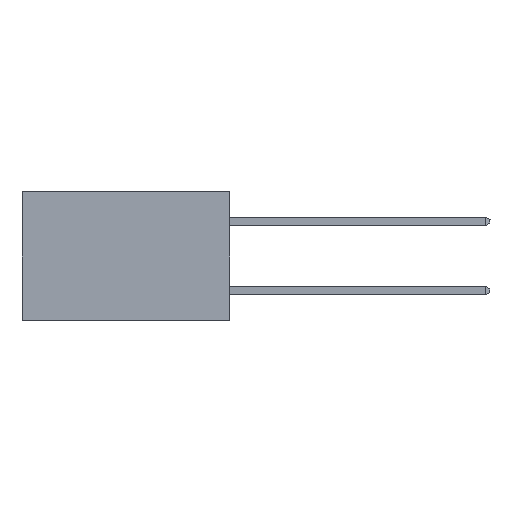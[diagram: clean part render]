
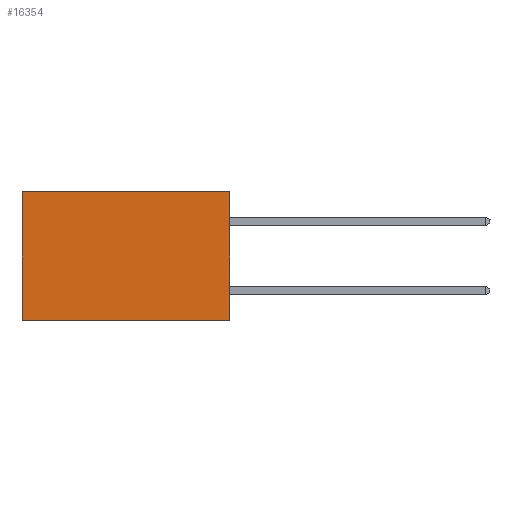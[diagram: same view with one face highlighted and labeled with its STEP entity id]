
A CAD part, left-side view. The second image highlights one B-rep face of the part: STEP entity #16354.
In plain terms, the highlighted planar face has unit normal (-1, 0, 0).
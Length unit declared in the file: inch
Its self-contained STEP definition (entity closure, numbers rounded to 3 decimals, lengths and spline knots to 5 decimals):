
#354 = CARTESIAN_POINT ( 'NONE',  ( 0.2615, 0., -0.37 ) ) ;
#1392 = FACE_OUTER_BOUND ( 'NONE', #18356, .T. ) ;
#1597 = VERTEX_POINT ( 'NONE', #5173 ) ;
#2340 = LINE ( 'NONE', #4180, #2395 ) ;
#2395 = VECTOR ( 'NONE', #3834, 39.37008 ) ;
#3674 = DIRECTION ( 'NONE',  ( 0., 0., -1. ) ) ;
#3834 = DIRECTION ( 'NONE',  ( 0., 0., -1. ) ) ;
#4180 = CARTESIAN_POINT ( 'NONE',  ( 0.2615, 0., -0.37 ) ) ;
#5068 = CARTESIAN_POINT ( 'NONE',  ( 0.2615, 0.6, -0.37 ) ) ;
#5173 = CARTESIAN_POINT ( 'NONE',  ( 0.2615, 0., -0.37 ) ) ;
#7219 = AXIS2_PLACEMENT_3D ( 'NONE', #8432, #11876, #11768 ) ;
#7254 = LINE ( 'NONE', #20901, #11094 ) ;
#8432 = CARTESIAN_POINT ( 'NONE',  ( 0.2615, 0., -0.37 ) ) ;
#8783 = EDGE_CURVE ( 'NONE', #10964, #18353, #7254, .T. ) ;
#9097 = LINE ( 'NONE', #354, #11551 ) ;
#10845 = CARTESIAN_POINT ( 'NONE',  ( 0.2615, 0., 0. ) ) ;
#10964 = VERTEX_POINT ( 'NONE', #17326 ) ;
#11094 = VECTOR ( 'NONE', #3674, 39.37008 ) ;
#11463 = ORIENTED_EDGE ( 'NONE', *, *, #13943, .T. ) ;
#11514 = ORIENTED_EDGE ( 'NONE', *, *, #13380, .F. ) ;
#11551 = VECTOR ( 'NONE', #14171, 39.37008 ) ;
#11586 = CARTESIAN_POINT ( 'NONE',  ( 0.2615, 0., 0. ) ) ;
#11768 = DIRECTION ( 'NONE',  ( 0., 0., -1. ) ) ;
#11876 = DIRECTION ( 'NONE',  ( 1., 0., 0. ) ) ;
#11877 = ORIENTED_EDGE ( 'NONE', *, *, #8783, .T. ) ;
#12514 = ORIENTED_EDGE ( 'NONE', *, *, #12820, .F. ) ;
#12820 = EDGE_CURVE ( 'NONE', #19770, #1597, #2340, .T. ) ;
#13380 = EDGE_CURVE ( 'NONE', #1597, #18353, #9097, .T. ) ;
#13943 = EDGE_CURVE ( 'NONE', #19770, #10964, #14830, .T. ) ;
#13950 = PLANE ( 'NONE',  #7219 ) ;
#14171 = DIRECTION ( 'NONE',  ( 0., 1., 0. ) ) ;
#14830 = LINE ( 'NONE', #11586, #15969 ) ;
#15969 = VECTOR ( 'NONE', #21796, 39.37008 ) ;
#16354 = ADVANCED_FACE ( 'NONE', ( #1392 ), #13950, .F. ) ;
#17326 = CARTESIAN_POINT ( 'NONE',  ( 0.2615, 0.6, 0. ) ) ;
#18353 = VERTEX_POINT ( 'NONE', #5068 ) ;
#18356 = EDGE_LOOP ( 'NONE', ( #11877, #11514, #12514, #11463 ) ) ;
#19770 = VERTEX_POINT ( 'NONE', #10845 ) ;
#20901 = CARTESIAN_POINT ( 'NONE',  ( 0.2615, 0.6, -0.37 ) ) ;
#21796 = DIRECTION ( 'NONE',  ( 0., 1., 0. ) ) ;
